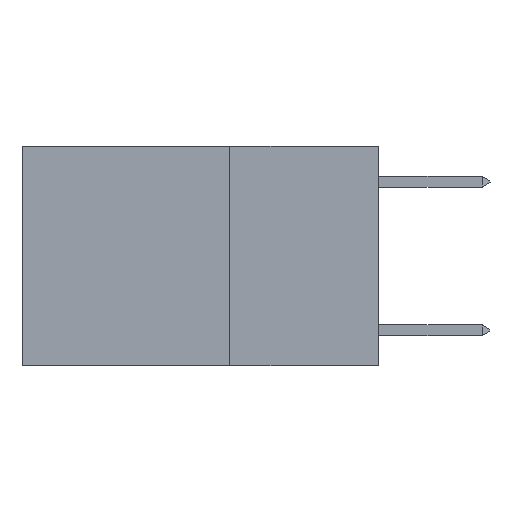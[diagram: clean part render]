
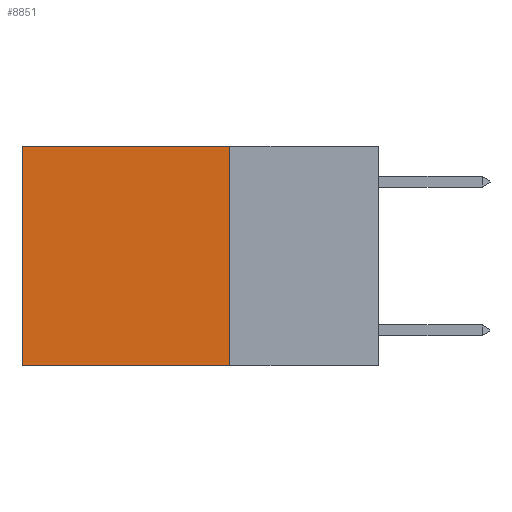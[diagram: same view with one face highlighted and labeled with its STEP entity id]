
A CAD part, left-side view. The second image highlights one B-rep face of the part: STEP entity #8851.
In plain terms, the highlighted planar face has unit normal (-1, 0, 0).
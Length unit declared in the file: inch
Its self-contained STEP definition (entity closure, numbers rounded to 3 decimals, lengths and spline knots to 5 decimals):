
#18 = DIRECTION ( 'NONE',  ( 0., 1., 0. ) ) ;
#351 = EDGE_LOOP ( 'NONE', ( #887, #6201, #1487, #4923 ) ) ;
#354 = LINE ( 'NONE', #5332, #4412 ) ;
#442 = DIRECTION ( 'NONE',  ( 0., 1., 0. ) ) ;
#581 = EDGE_CURVE ( 'NONE', #7912, #2651, #354, .T. ) ;
#887 = ORIENTED_EDGE ( 'NONE', *, *, #581, .T. ) ;
#1487 = ORIENTED_EDGE ( 'NONE', *, *, #5609, .F. ) ;
#1537 = DIRECTION ( 'NONE',  ( 1., 0., 0. ) ) ;
#2119 = DIRECTION ( 'NONE',  ( 0., 0., -1. ) ) ;
#2167 = AXIS2_PLACEMENT_3D ( 'NONE', #3927, #1537, #7116 ) ;
#2446 = LINE ( 'NONE', #7999, #4605 ) ;
#2613 = DIRECTION ( 'NONE',  ( 0., 0., -1. ) ) ;
#2651 = VERTEX_POINT ( 'NONE', #4808 ) ;
#3881 = EDGE_CURVE ( 'NONE', #5172, #2651, #2446, .T. ) ;
#3927 = CARTESIAN_POINT ( 'NONE',  ( 0.2625, 0.25, 0. ) ) ;
#4073 = LINE ( 'NONE', #9935, #10295 ) ;
#4412 = VECTOR ( 'NONE', #2119, 39.37008 ) ;
#4489 = VECTOR ( 'NONE', #442, 39.37008 ) ;
#4605 = VECTOR ( 'NONE', #18, 39.37008 ) ;
#4733 = PLANE ( 'NONE',  #2167 ) ;
#4808 = CARTESIAN_POINT ( 'NONE',  ( 0.2625, 0.6, -0.37 ) ) ;
#4923 = ORIENTED_EDGE ( 'NONE', *, *, #8031, .T. ) ;
#5172 = VERTEX_POINT ( 'NONE', #7637 ) ;
#5332 = CARTESIAN_POINT ( 'NONE',  ( 0.2625, 0.6, 0. ) ) ;
#5609 = EDGE_CURVE ( 'NONE', #8392, #5172, #4073, .T. ) ;
#6201 = ORIENTED_EDGE ( 'NONE', *, *, #3881, .F. ) ;
#6591 = LINE ( 'NONE', #10172, #4489 ) ;
#7116 = DIRECTION ( 'NONE',  ( 0., 0., -1. ) ) ;
#7433 = CARTESIAN_POINT ( 'NONE',  ( 0.2625, 0.25, 0. ) ) ;
#7637 = CARTESIAN_POINT ( 'NONE',  ( 0.2625, 0.25, -0.37 ) ) ;
#7912 = VERTEX_POINT ( 'NONE', #9228 ) ;
#7999 = CARTESIAN_POINT ( 'NONE',  ( 0.2625, 0.25, -0.37 ) ) ;
#8031 = EDGE_CURVE ( 'NONE', #8392, #7912, #6591, .T. ) ;
#8311 = FACE_OUTER_BOUND ( 'NONE', #351, .T. ) ;
#8392 = VERTEX_POINT ( 'NONE', #7433 ) ;
#8851 = ADVANCED_FACE ( 'NONE', ( #8311 ), #4733, .F. ) ;
#9228 = CARTESIAN_POINT ( 'NONE',  ( 0.2625, 0.6, 0. ) ) ;
#9935 = CARTESIAN_POINT ( 'NONE',  ( 0.2625, 0.25, 0. ) ) ;
#10172 = CARTESIAN_POINT ( 'NONE',  ( 0.2625, 0.25, 0. ) ) ;
#10295 = VECTOR ( 'NONE', #2613, 39.37008 ) ;
